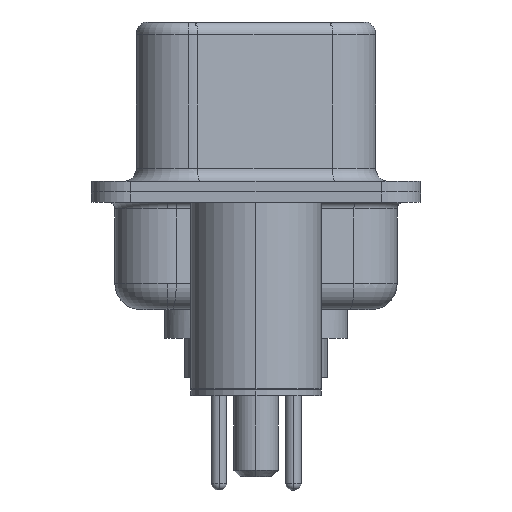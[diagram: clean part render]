
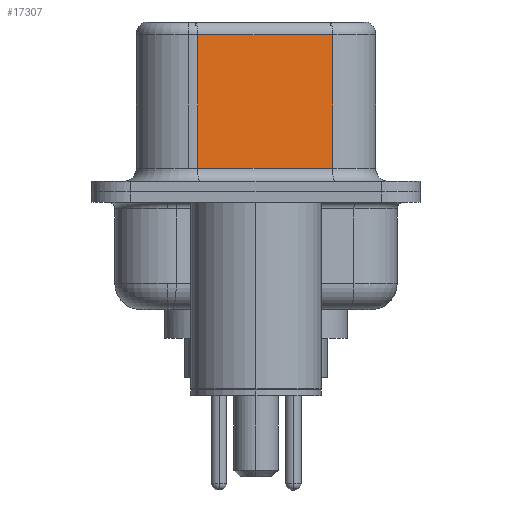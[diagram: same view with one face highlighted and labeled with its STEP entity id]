
A CAD part, left-side view. The second image highlights one B-rep face of the part: STEP entity #17307.
In plain terms, the highlighted planar face has unit normal (-0.985, -0.174, 0).
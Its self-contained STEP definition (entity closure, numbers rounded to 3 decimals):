
#64 = CARTESIAN_POINT ( 'NONE',  ( 3.67, 2.233, 6.52 ) ) ;
#253 = LINE ( 'NONE', #10674, #19652 ) ;
#497 = DIRECTION ( 'NONE',  ( 0.985, 0.174, 0. ) ) ;
#1007 = VERTEX_POINT ( 'NONE', #13038 ) ;
#1459 = DIRECTION ( 'NONE',  ( 0., 0., -1. ) ) ;
#1483 = DIRECTION ( 'NONE',  ( -0.174, 0.985, 0. ) ) ;
#1720 = VERTEX_POINT ( 'NONE', #4474 ) ;
#2076 = CARTESIAN_POINT ( 'NONE',  ( 4.58, -2.927, 6.52 ) ) ;
#2283 = FACE_OUTER_BOUND ( 'NONE', #6605, .T. ) ;
#3700 = DIRECTION ( 'NONE',  ( 0., 0., -1. ) ) ;
#4220 = VERTEX_POINT ( 'NONE', #9216 ) ;
#4312 = DIRECTION ( 'NONE',  ( 0.174, -0.985, 0. ) ) ;
#4413 = VECTOR ( 'NONE', #4312, 1000. ) ;
#4474 = CARTESIAN_POINT ( 'NONE',  ( 4.58, -2.927, 6.02 ) ) ;
#4957 = VECTOR ( 'NONE', #3700, 1000. ) ;
#5118 = EDGE_CURVE ( 'NONE', #1720, #1007, #18371, .T. ) ;
#6605 = EDGE_LOOP ( 'NONE', ( #12761, #10340, #8837, #9926 ) ) ;
#6885 = EDGE_CURVE ( 'NONE', #4220, #1007, #17643, .T. ) ;
#7277 = AXIS2_PLACEMENT_3D ( 'NONE', #11358, #497, #11287 ) ;
#8837 = ORIENTED_EDGE ( 'NONE', *, *, #18530, .T. ) ;
#9216 = CARTESIAN_POINT ( 'NONE',  ( 3.67, 2.233, 0.9 ) ) ;
#9903 = CARTESIAN_POINT ( 'NONE',  ( 4.58, -2.927, 0.9 ) ) ;
#9926 = ORIENTED_EDGE ( 'NONE', *, *, #6885, .T. ) ;
#10177 = EDGE_CURVE ( 'NONE', #1720, #16908, #253, .T. ) ;
#10340 = ORIENTED_EDGE ( 'NONE', *, *, #10177, .T. ) ;
#10674 = CARTESIAN_POINT ( 'NONE',  ( 4.58, -2.927, 6.02 ) ) ;
#11287 = DIRECTION ( 'NONE',  ( -0.174, 0.985, 0. ) ) ;
#11358 = CARTESIAN_POINT ( 'NONE',  ( 4.58, -2.927, 6.52 ) ) ;
#12761 = ORIENTED_EDGE ( 'NONE', *, *, #5118, .F. ) ;
#13038 = CARTESIAN_POINT ( 'NONE',  ( 4.58, -2.927, 0.9 ) ) ;
#16640 = LINE ( 'NONE', #64, #17615 ) ;
#16908 = VERTEX_POINT ( 'NONE', #19057 ) ;
#17307 = ADVANCED_FACE ( 'NONE', ( #2283 ), #17324, .F. ) ;
#17324 = PLANE ( 'NONE',  #7277 ) ;
#17615 = VECTOR ( 'NONE', #1459, 1000. ) ;
#17643 = LINE ( 'NONE', #9903, #4413 ) ;
#18371 = LINE ( 'NONE', #2076, #4957 ) ;
#18530 = EDGE_CURVE ( 'NONE', #16908, #4220, #16640, .T. ) ;
#19057 = CARTESIAN_POINT ( 'NONE',  ( 3.67, 2.233, 6.02 ) ) ;
#19652 = VECTOR ( 'NONE', #1483, 1000. ) ;
